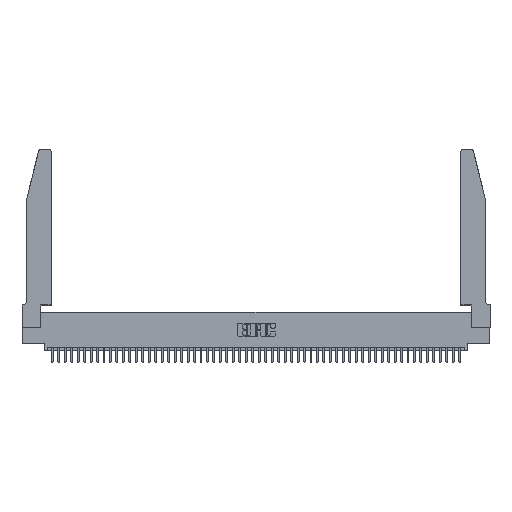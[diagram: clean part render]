
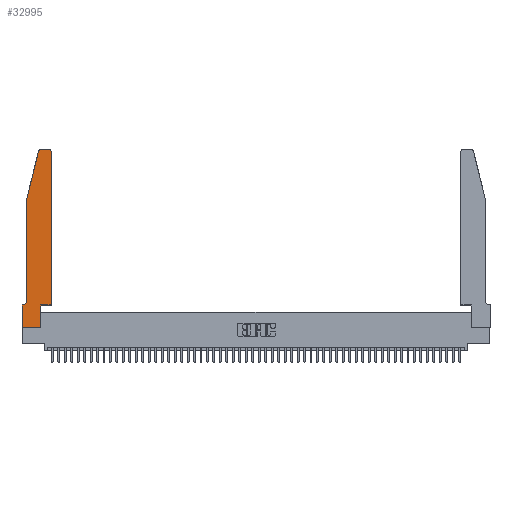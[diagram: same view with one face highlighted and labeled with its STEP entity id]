
A CAD part, top view. The second image highlights one B-rep face of the part: STEP entity #32995.
In plain terms, the highlighted planar face has unit normal (0, 0, 1).
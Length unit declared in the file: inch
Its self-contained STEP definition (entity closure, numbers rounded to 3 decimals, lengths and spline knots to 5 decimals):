
#650 = VECTOR ( 'NONE', #32371, 39.37008 ) ;
#1213 = VERTEX_POINT ( 'NONE', #36772 ) ;
#1619 = DIRECTION ( 'NONE',  ( -1., 0., 0. ) ) ;
#1625 = DIRECTION ( 'NONE',  ( 0., -1., 0. ) ) ;
#1693 = CARTESIAN_POINT ( 'NONE',  ( 0.4505, 0.35, 0.37 ) ) ;
#1749 = EDGE_CURVE ( 'NONE', #48536, #9952, #32908, .T. ) ;
#3378 = CARTESIAN_POINT ( 'NONE',  ( 0.2865, 0.35, 0.37 ) ) ;
#4548 = CARTESIAN_POINT ( 'NONE',  ( 0.0755, 0.35, 0.37 ) ) ;
#4576 = ORIENTED_EDGE ( 'NONE', *, *, #15255, .T. ) ;
#5318 = ORIENTED_EDGE ( 'NONE', *, *, #43974, .T. ) ;
#5454 = VECTOR ( 'NONE', #8643, 39.37008 ) ;
#5548 = CARTESIAN_POINT ( 'NONE',  ( 0.2605, 2.75, 0.37 ) ) ;
#5941 = DIRECTION ( 'NONE',  ( 0., 0., -1. ) ) ;
#6531 = CARTESIAN_POINT ( 'NONE',  ( 0.25487, 2.72718, 0.37 ) ) ;
#6673 = CARTESIAN_POINT ( 'NONE',  ( 0.0055, 0.35, 0.37 ) ) ;
#7269 = VECTOR ( 'NONE', #1619, 39.37008 ) ;
#7526 = VECTOR ( 'NONE', #14232, 39.37008 ) ;
#7811 = VECTOR ( 'NONE', #23544, 39.37008 ) ;
#8253 = AXIS2_PLACEMENT_3D ( 'NONE', #21220, #49448, #25238 ) ;
#8306 = VERTEX_POINT ( 'NONE', #37803 ) ;
#8542 = EDGE_CURVE ( 'NONE', #1213, #48402, #27999, .T. ) ;
#8643 = DIRECTION ( 'NONE',  ( -1., 0., 0. ) ) ;
#8907 = ORIENTED_EDGE ( 'NONE', *, *, #35384, .T. ) ;
#9173 = VERTEX_POINT ( 'NONE', #16399 ) ;
#9480 = VERTEX_POINT ( 'NONE', #39422 ) ;
#9952 = VERTEX_POINT ( 'NONE', #13477 ) ;
#10154 = CARTESIAN_POINT ( 'NONE',  ( 0., 0., 0.37 ) ) ;
#10343 = ORIENTED_EDGE ( 'NONE', *, *, #1749, .T. ) ;
#10536 = PLANE ( 'NONE',  #39983 ) ;
#10679 = CIRCLE ( 'NONE', #44904, 0.07 ) ;
#12280 = CARTESIAN_POINT ( 'NONE',  ( 0.0755, 2., 0.37 ) ) ;
#13008 = FACE_OUTER_BOUND ( 'NONE', #38356, .T. ) ;
#13459 = CARTESIAN_POINT ( 'NONE',  ( 0., 0., 0.37 ) ) ;
#13477 = CARTESIAN_POINT ( 'NONE',  ( 0.0755, 2., 0.37 ) ) ;
#13996 = ORIENTED_EDGE ( 'NONE', *, *, #39491, .T. ) ;
#14029 = EDGE_CURVE ( 'NONE', #46283, #1213, #39632, .T. ) ;
#14232 = DIRECTION ( 'NONE',  ( 1., 0., 0. ) ) ;
#14606 = DIRECTION ( 'NONE',  ( 1., 0., 0. ) ) ;
#15255 = EDGE_CURVE ( 'NONE', #9173, #48536, #47174, .T. ) ;
#15620 = EDGE_CURVE ( 'NONE', #50611, #8306, #16180, .T. ) ;
#16180 = LINE ( 'NONE', #4548, #5454 ) ;
#16240 = ORIENTED_EDGE ( 'NONE', *, *, #21879, .T. ) ;
#16399 = CARTESIAN_POINT ( 'NONE',  ( 0.284, 2.75, 0.37 ) ) ;
#17775 = CARTESIAN_POINT ( 'NONE',  ( 0., 0., 0.37 ) ) ;
#19728 = LINE ( 'NONE', #46777, #29161 ) ;
#21220 = CARTESIAN_POINT ( 'NONE',  ( 0.4205, 2.72, 0.37 ) ) ;
#21360 = CARTESIAN_POINT ( 'NONE',  ( 0.4505, 2.72, 0.37 ) ) ;
#21841 = DIRECTION ( 'NONE',  ( 0., -1., 0. ) ) ;
#21879 = EDGE_CURVE ( 'NONE', #25935, #9480, #50327, .T. ) ;
#22411 = CARTESIAN_POINT ( 'NONE',  ( 0.284, 2.72, 0.37 ) ) ;
#22615 = DIRECTION ( 'NONE',  ( 0., 1., 0. ) ) ;
#23270 = EDGE_CURVE ( 'NONE', #9480, #9173, #28713, .T. ) ;
#23544 = DIRECTION ( 'NONE',  ( 0., 1., 0. ) ) ;
#23833 = ORIENTED_EDGE ( 'NONE', *, *, #8542, .T. ) ;
#25238 = DIRECTION ( 'NONE',  ( 1., 0., 0. ) ) ;
#25336 = VERTEX_POINT ( 'NONE', #36865 ) ;
#25854 = VECTOR ( 'NONE', #21841, 39.37008 ) ;
#25935 = VERTEX_POINT ( 'NONE', #21360 ) ;
#26442 = DIRECTION ( 'NONE',  ( 1., 0., 0. ) ) ;
#27999 = LINE ( 'NONE', #3378, #7811 ) ;
#28579 = VECTOR ( 'NONE', #29977, 39.37008 ) ;
#28594 = ORIENTED_EDGE ( 'NONE', *, *, #41569, .T. ) ;
#28713 = LINE ( 'NONE', #5548, #7269 ) ;
#29161 = VECTOR ( 'NONE', #22615, 39.37008 ) ;
#29977 = DIRECTION ( 'NONE',  ( 1., 0., 0. ) ) ;
#30091 = CARTESIAN_POINT ( 'NONE',  ( 0.0055, 0.42, 0.37 ) ) ;
#32371 = DIRECTION ( 'NONE',  ( -0.239, -0.971, 0. ) ) ;
#32383 = ORIENTED_EDGE ( 'NONE', *, *, #37614, .T. ) ;
#32908 = LINE ( 'NONE', #12280, #650 ) ;
#32995 = ADVANCED_FACE ( 'NONE', ( #13008 ), #10536, .T. ) ;
#33096 = ORIENTED_EDGE ( 'NONE', *, *, #15620, .T. ) ;
#34128 = DIRECTION ( 'NONE',  ( -1., 0., 0. ) ) ;
#34457 = VECTOR ( 'NONE', #1625, 39.37008 ) ;
#35384 = EDGE_CURVE ( 'NONE', #48402, #25336, #37991, .T. ) ;
#36772 = CARTESIAN_POINT ( 'NONE',  ( 0.2865, 0., 0.37 ) ) ;
#36865 = CARTESIAN_POINT ( 'NONE',  ( 0.4505, 0.35, 0.37 ) ) ;
#37614 = EDGE_CURVE ( 'NONE', #42637, #50611, #10679, .T. ) ;
#37803 = CARTESIAN_POINT ( 'NONE',  ( 0., 0.35, 0.37 ) ) ;
#37870 = CARTESIAN_POINT ( 'NONE',  ( 0.2865, 0.35, 0.37 ) ) ;
#37991 = LINE ( 'NONE', #1693, #28579 ) ;
#38356 = EDGE_LOOP ( 'NONE', ( #46781, #4576, #10343, #28594, #32383, #33096, #13996, #47354, #23833, #8907, #5318, #16240 ) ) ;
#38693 = DIRECTION ( 'NONE',  ( 0., 0., 1. ) ) ;
#39422 = CARTESIAN_POINT ( 'NONE',  ( 0.4205, 2.75, 0.37 ) ) ;
#39491 = EDGE_CURVE ( 'NONE', #8306, #46283, #47336, .T. ) ;
#39632 = LINE ( 'NONE', #10154, #7526 ) ;
#39983 = AXIS2_PLACEMENT_3D ( 'NONE', #50744, #38693, #14606 ) ;
#41569 = EDGE_CURVE ( 'NONE', #9952, #42637, #45203, .T. ) ;
#42637 = VERTEX_POINT ( 'NONE', #48332 ) ;
#43974 = EDGE_CURVE ( 'NONE', #25336, #25935, #19728, .T. ) ;
#44904 = AXIS2_PLACEMENT_3D ( 'NONE', #30091, #5941, #34128 ) ;
#45203 = LINE ( 'NONE', #50005, #34457 ) ;
#45554 = AXIS2_PLACEMENT_3D ( 'NONE', #22411, #50604, #26442 ) ;
#46283 = VERTEX_POINT ( 'NONE', #13459 ) ;
#46777 = CARTESIAN_POINT ( 'NONE',  ( 0.4505, 0.35, 0.37 ) ) ;
#46781 = ORIENTED_EDGE ( 'NONE', *, *, #23270, .T. ) ;
#47174 = CIRCLE ( 'NONE', #45554, 0.03 ) ;
#47336 = LINE ( 'NONE', #17775, #25854 ) ;
#47354 = ORIENTED_EDGE ( 'NONE', *, *, #14029, .T. ) ;
#48332 = CARTESIAN_POINT ( 'NONE',  ( 0.0755, 0.42, 0.37 ) ) ;
#48402 = VERTEX_POINT ( 'NONE', #37870 ) ;
#48536 = VERTEX_POINT ( 'NONE', #6531 ) ;
#49448 = DIRECTION ( 'NONE',  ( 0., 0., 1. ) ) ;
#50005 = CARTESIAN_POINT ( 'NONE',  ( 0.0755, 2., 0.37 ) ) ;
#50327 = CIRCLE ( 'NONE', #8253, 0.03 ) ;
#50604 = DIRECTION ( 'NONE',  ( 0., 0., 1. ) ) ;
#50611 = VERTEX_POINT ( 'NONE', #6673 ) ;
#50744 = CARTESIAN_POINT ( 'NONE',  ( 0., 0.35, 0.37 ) ) ;
